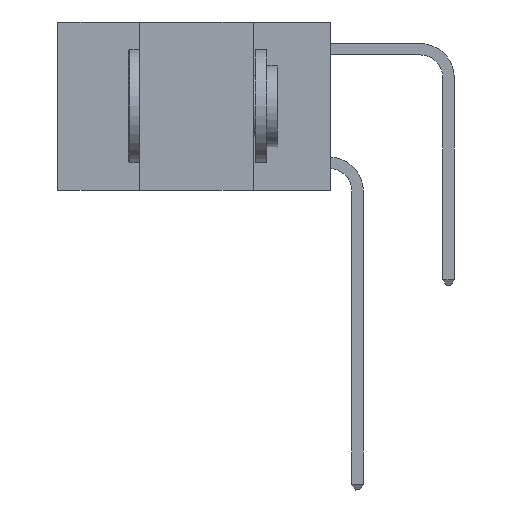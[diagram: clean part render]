
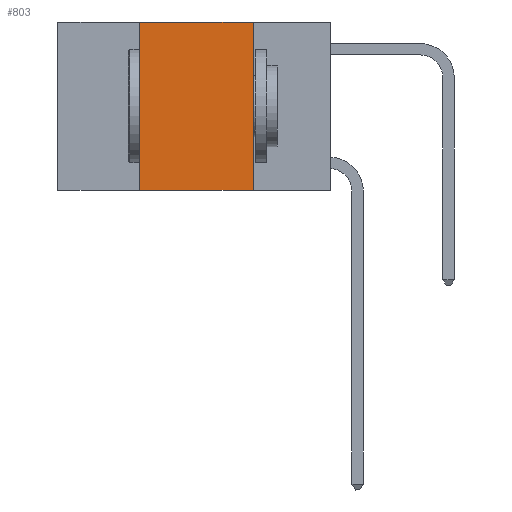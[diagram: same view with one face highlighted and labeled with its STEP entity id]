
A CAD part, left-side view. The second image highlights one B-rep face of the part: STEP entity #803.
In plain terms, the highlighted planar face has unit normal (-1, 0, 0).
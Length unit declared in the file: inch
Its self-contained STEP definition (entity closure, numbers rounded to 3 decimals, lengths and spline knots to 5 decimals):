
#803 = ADVANCED_FACE ( 'NONE', ( #1819 ), #7657, .F. ) ;
#1569 = CARTESIAN_POINT ( 'NONE',  ( 0., 0.6, -0.37 ) ) ;
#1819 = FACE_OUTER_BOUND ( 'NONE', #10603, .T. ) ;
#2010 = ORIENTED_EDGE ( 'NONE', *, *, #5155, .F. ) ;
#2248 = EDGE_CURVE ( 'NONE', #10487, #5902, #6844, .T. ) ;
#2351 = DIRECTION ( 'NONE',  ( 0., -1., 0. ) ) ;
#2815 = EDGE_CURVE ( 'NONE', #3733, #10487, #5658, .T. ) ;
#2936 = CARTESIAN_POINT ( 'NONE',  ( 0., 0.6, 0. ) ) ;
#3730 = DIRECTION ( 'NONE',  ( 0., 0., -1. ) ) ;
#3733 = VERTEX_POINT ( 'NONE', #9843 ) ;
#3867 = CARTESIAN_POINT ( 'NONE',  ( 0., 0.17, 0. ) ) ;
#4036 = AXIS2_PLACEMENT_3D ( 'NONE', #7711, #7550, #7420 ) ;
#4108 = VERTEX_POINT ( 'NONE', #12899 ) ;
#4904 = CARTESIAN_POINT ( 'NONE',  ( 0., 0.17, 0. ) ) ;
#5155 = EDGE_CURVE ( 'NONE', #4108, #3733, #16008, .T. ) ;
#5658 = LINE ( 'NONE', #2936, #11825 ) ;
#5902 = VERTEX_POINT ( 'NONE', #12324 ) ;
#6844 = LINE ( 'NONE', #3867, #9704 ) ;
#7420 = DIRECTION ( 'NONE',  ( 0., 0., -1. ) ) ;
#7550 = DIRECTION ( 'NONE',  ( 1., 0., 0. ) ) ;
#7657 = PLANE ( 'NONE',  #4036 ) ;
#7711 = CARTESIAN_POINT ( 'NONE',  ( 0., 0.6, 0. ) ) ;
#7846 = ORIENTED_EDGE ( 'NONE', *, *, #2248, .F. ) ;
#8580 = CARTESIAN_POINT ( 'NONE',  ( 0., 0.42, 0. ) ) ;
#9494 = VECTOR ( 'NONE', #9804, 39.37008 ) ;
#9704 = VECTOR ( 'NONE', #3730, 39.37008 ) ;
#9804 = DIRECTION ( 'NONE',  ( 0., 0., 1. ) ) ;
#9843 = CARTESIAN_POINT ( 'NONE',  ( 0., 0.42, 0. ) ) ;
#10001 = EDGE_CURVE ( 'NONE', #4108, #5902, #10494, .T. ) ;
#10487 = VERTEX_POINT ( 'NONE', #4904 ) ;
#10494 = LINE ( 'NONE', #1569, #10875 ) ;
#10603 = EDGE_LOOP ( 'NONE', ( #7846, #14349, #2010, #12259 ) ) ;
#10875 = VECTOR ( 'NONE', #12689, 39.37008 ) ;
#11825 = VECTOR ( 'NONE', #2351, 39.37008 ) ;
#12259 = ORIENTED_EDGE ( 'NONE', *, *, #10001, .T. ) ;
#12324 = CARTESIAN_POINT ( 'NONE',  ( 0., 0.17, -0.37 ) ) ;
#12689 = DIRECTION ( 'NONE',  ( 0., -1., 0. ) ) ;
#12899 = CARTESIAN_POINT ( 'NONE',  ( 0., 0.42, -0.37 ) ) ;
#14349 = ORIENTED_EDGE ( 'NONE', *, *, #2815, .F. ) ;
#16008 = LINE ( 'NONE', #8580, #9494 ) ;
